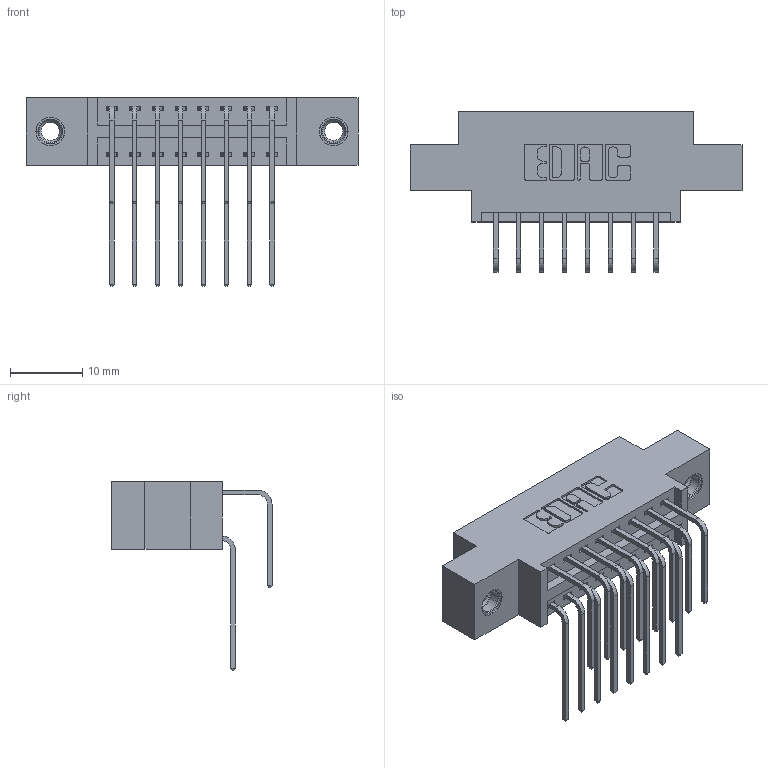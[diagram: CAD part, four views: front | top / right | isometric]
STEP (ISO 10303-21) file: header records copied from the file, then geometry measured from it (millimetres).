
FILE_DESCRIPTION (( 'STEP AP203' ), '1' );
FILE_NAME ('396-016-558-807.STEP', '2019-11-02T13:59:08', ( '' ), ( '' ), 'SwSTEP 2.0', 'SolidWorks 2016', '' );
FILE_SCHEMA (( 'CONFIG_CONTROL_DESIGN' ));
Length unit declared in the file: inch
Products named in the file (5): 396-016-558-807; 345-250-001_345-250-005-103; 345-292-001_558 Tail - 2; 345-292-001_558 559 Tail - 1; 346 Part_0.170 Offset - 0.156 Dia-TI
Assembly tree (19 placements, depth 2):
  396-016-558-807
    346 Part_0.170 Offset - 0.156 Dia-TI
    345-292-001_558 559 Tail - 1  x8
    345-292-001_558 Tail - 2  x8
    345-250-001_345-250-005-103  x2
Bounding box: 45.97 x 22.16 x 26.16 mm (x, y, z)
Volume: 4143.1 mm3; surface area: 5816.8 mm2
Topology: 19 solids, 19 shells, 1050 faces, 3053 edges, 2006 vertices
Faces by surface type: plane 704, cylinder 330, cone 12, torus 4
Entity records: 12900 total; most frequent: CARTESIAN_POINT 2210, ORIENTED_EDGE 2086, DIRECTION 1997, EDGE_CURVE 1043, LINE 819, VECTOR 819, VERTEX_POINT 688, AXIS2_PLACEMENT_3D 589
